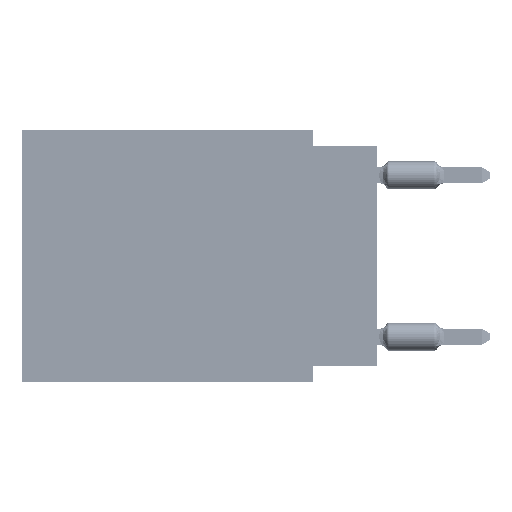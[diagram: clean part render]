
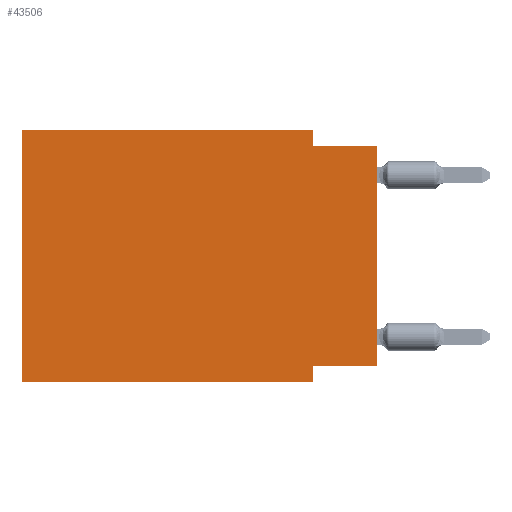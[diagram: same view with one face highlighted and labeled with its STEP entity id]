
A CAD part, left-side view. The second image highlights one B-rep face of the part: STEP entity #43506.
In plain terms, the highlighted planar face has unit normal (-1, 0, 0).
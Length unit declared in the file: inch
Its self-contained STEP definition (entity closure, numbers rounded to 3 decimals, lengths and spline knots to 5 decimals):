
#8 = ORIENTED_EDGE ( 'NONE', *, *, #29988, .F. ) ;
#160 = EDGE_CURVE ( 'NONE', #21846, #71456, #30832, .T. ) ;
#1071 = EDGE_CURVE ( 'NONE', #14515, #29453, #33141, .T. ) ;
#1657 = CARTESIAN_POINT ( 'NONE',  ( 0., 0., 0. ) ) ;
#5803 = LINE ( 'NONE', #56205, #10860 ) ;
#6381 = VECTOR ( 'NONE', #20555, 39.37008 ) ;
#7225 = DIRECTION ( 'NONE',  ( 0., -1., 0. ) ) ;
#10633 = FACE_OUTER_BOUND ( 'NONE', #16403, .T. ) ;
#10860 = VECTOR ( 'NONE', #39541, 39.37008 ) ;
#13671 = CARTESIAN_POINT ( 'NONE',  ( 0., 0.1, -0.39 ) ) ;
#14515 = VERTEX_POINT ( 'NONE', #18132 ) ;
#14950 = VERTEX_POINT ( 'NONE', #35113 ) ;
#15819 = PLANE ( 'NONE',  #70205 ) ;
#16010 = CARTESIAN_POINT ( 'NONE',  ( 0., 0., -0.025 ) ) ;
#16403 = EDGE_LOOP ( 'NONE', ( #44305, #8, #24323, #33468, #64175, #64086, #60328, #17260 ) ) ;
#17260 = ORIENTED_EDGE ( 'NONE', *, *, #43801, .F. ) ;
#17534 = EDGE_CURVE ( 'NONE', #33354, #48256, #58708, .T. ) ;
#18109 = VECTOR ( 'NONE', #34120, 39.37008 ) ;
#18132 = CARTESIAN_POINT ( 'NONE',  ( 0., 0.55, -0.39 ) ) ;
#19373 = DIRECTION ( 'NONE',  ( 0., 0., -1. ) ) ;
#19427 = CARTESIAN_POINT ( 'NONE',  ( 0., 0.55, -0.39 ) ) ;
#19438 = VECTOR ( 'NONE', #47239, 39.37008 ) ;
#20555 = DIRECTION ( 'NONE',  ( 0., 1., 0. ) ) ;
#21846 = VERTEX_POINT ( 'NONE', #67701 ) ;
#22039 = CARTESIAN_POINT ( 'NONE',  ( 0., 0.55, 0. ) ) ;
#24323 = ORIENTED_EDGE ( 'NONE', *, *, #160, .F. ) ;
#24627 = EDGE_CURVE ( 'NONE', #14515, #61621, #64268, .T. ) ;
#26284 = CARTESIAN_POINT ( 'NONE',  ( 0., 0., -0.365 ) ) ;
#28405 = DIRECTION ( 'NONE',  ( 0., 0., -1. ) ) ;
#29453 = VERTEX_POINT ( 'NONE', #38142 ) ;
#29988 = EDGE_CURVE ( 'NONE', #71456, #48256, #5803, .T. ) ;
#30832 = LINE ( 'NONE', #56552, #41536 ) ;
#31226 = CARTESIAN_POINT ( 'NONE',  ( 0., 0.1, -0.39 ) ) ;
#32348 = VECTOR ( 'NONE', #54277, 39.37008 ) ;
#33141 = LINE ( 'NONE', #22039, #32348 ) ;
#33354 = VERTEX_POINT ( 'NONE', #26284 ) ;
#33468 = ORIENTED_EDGE ( 'NONE', *, *, #65115, .F. ) ;
#33972 = CARTESIAN_POINT ( 'NONE',  ( 0., 0.55, 0. ) ) ;
#34120 = DIRECTION ( 'NONE',  ( 0., -1., 0. ) ) ;
#35113 = CARTESIAN_POINT ( 'NONE',  ( 0., 0.1, -0.365 ) ) ;
#38142 = CARTESIAN_POINT ( 'NONE',  ( 0., 0.55, 0. ) ) ;
#39168 = DIRECTION ( 'NONE',  ( 1., 0., 0. ) ) ;
#39251 = CARTESIAN_POINT ( 'NONE',  ( 0., 0.1, -0.025 ) ) ;
#39541 = DIRECTION ( 'NONE',  ( 0., -1., 0. ) ) ;
#39687 = CARTESIAN_POINT ( 'NONE',  ( 0., 0.55, 0. ) ) ;
#41536 = VECTOR ( 'NONE', #69755, 39.37008 ) ;
#43506 = ADVANCED_FACE ( 'NONE', ( #10633 ), #15819, .F. ) ;
#43801 = EDGE_CURVE ( 'NONE', #33354, #14950, #70950, .T. ) ;
#44305 = ORIENTED_EDGE ( 'NONE', *, *, #17534, .T. ) ;
#46333 = LINE ( 'NONE', #39687, #18109 ) ;
#46427 = EDGE_CURVE ( 'NONE', #14950, #61621, #70136, .T. ) ;
#47239 = DIRECTION ( 'NONE',  ( 0., 0., 1. ) ) ;
#48256 = VERTEX_POINT ( 'NONE', #16010 ) ;
#54277 = DIRECTION ( 'NONE',  ( 0., 0., 1. ) ) ;
#56205 = CARTESIAN_POINT ( 'NONE',  ( 0., 0., -0.025 ) ) ;
#56552 = CARTESIAN_POINT ( 'NONE',  ( 0., 0.1, 0. ) ) ;
#58708 = LINE ( 'NONE', #1657, #19438 ) ;
#60328 = ORIENTED_EDGE ( 'NONE', *, *, #46427, .F. ) ;
#60562 = CARTESIAN_POINT ( 'NONE',  ( 0., 0., -0.365 ) ) ;
#61621 = VERTEX_POINT ( 'NONE', #13671 ) ;
#64086 = ORIENTED_EDGE ( 'NONE', *, *, #24627, .T. ) ;
#64175 = ORIENTED_EDGE ( 'NONE', *, *, #1071, .F. ) ;
#64268 = LINE ( 'NONE', #19427, #66116 ) ;
#65115 = EDGE_CURVE ( 'NONE', #29453, #21846, #46333, .T. ) ;
#66116 = VECTOR ( 'NONE', #7225, 39.37008 ) ;
#67119 = VECTOR ( 'NONE', #19373, 39.37008 ) ;
#67701 = CARTESIAN_POINT ( 'NONE',  ( 0., 0.1, 0. ) ) ;
#69755 = DIRECTION ( 'NONE',  ( 0., 0., -1. ) ) ;
#70136 = LINE ( 'NONE', #31226, #67119 ) ;
#70205 = AXIS2_PLACEMENT_3D ( 'NONE', #33972, #39168, #28405 ) ;
#70950 = LINE ( 'NONE', #60562, #6381 ) ;
#71456 = VERTEX_POINT ( 'NONE', #39251 ) ;
